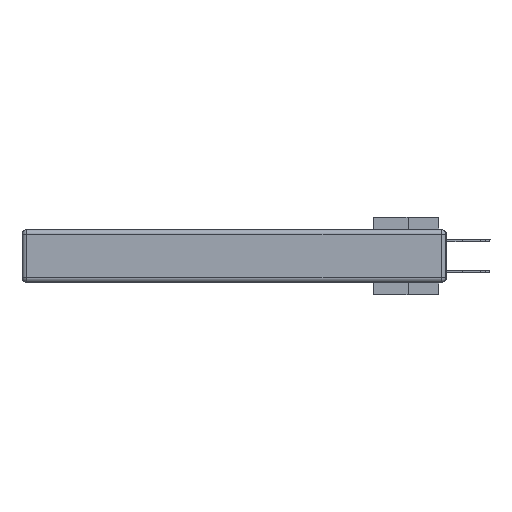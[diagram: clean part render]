
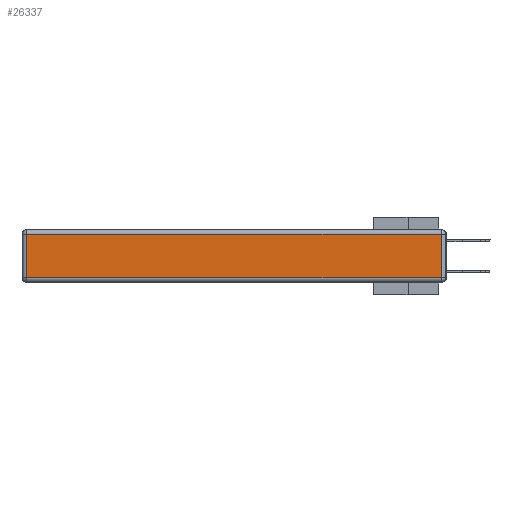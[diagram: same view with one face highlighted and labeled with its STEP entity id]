
A CAD part, left-side view. The second image highlights one B-rep face of the part: STEP entity #26337.
In plain terms, the highlighted planar face has unit normal (-1, 0, 0).
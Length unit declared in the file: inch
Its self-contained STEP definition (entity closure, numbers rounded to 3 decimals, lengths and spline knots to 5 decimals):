
#315 = CARTESIAN_POINT ( 'NONE',  ( 0., 2.72, -0.03 ) ) ;
#1589 = CARTESIAN_POINT ( 'NONE',  ( 0., 0.03, -0.03 ) ) ;
#2590 = ORIENTED_EDGE ( 'NONE', *, *, #18091, .T. ) ;
#4384 = CARTESIAN_POINT ( 'NONE',  ( 0., 0., -0.313 ) ) ;
#4401 = VECTOR ( 'NONE', #8673, 39.37008 ) ;
#5197 = CARTESIAN_POINT ( 'NONE',  ( 0., 0.03, -0.343 ) ) ;
#5312 = DIRECTION ( 'NONE',  ( 0., 1., 0. ) ) ;
#6022 = VECTOR ( 'NONE', #21128, 39.37008 ) ;
#6031 = LINE ( 'NONE', #25385, #21256 ) ;
#6754 = CARTESIAN_POINT ( 'NONE',  ( 0., 0.03, -0.313 ) ) ;
#6885 = LINE ( 'NONE', #4384, #4401 ) ;
#8673 = DIRECTION ( 'NONE',  ( 0., -1., 0. ) ) ;
#8689 = VECTOR ( 'NONE', #17962, 39.37008 ) ;
#9692 = CARTESIAN_POINT ( 'NONE',  ( 0., 0., -0.343 ) ) ;
#10976 = ORIENTED_EDGE ( 'NONE', *, *, #23696, .T. ) ;
#11354 = EDGE_LOOP ( 'NONE', ( #21971, #10976, #28337, #2590 ) ) ;
#13996 = PLANE ( 'NONE',  #22087 ) ;
#15625 = LINE ( 'NONE', #5197, #6022 ) ;
#16360 = DIRECTION ( 'NONE',  ( 0., 0., 1. ) ) ;
#16984 = CARTESIAN_POINT ( 'NONE',  ( 0., 2.72, -0.313 ) ) ;
#17520 = EDGE_CURVE ( 'NONE', #25923, #25482, #6885, .T. ) ;
#17962 = DIRECTION ( 'NONE',  ( 0., 0., -1. ) ) ;
#18091 = EDGE_CURVE ( 'NONE', #28902, #25923, #20392, .T. ) ;
#19339 = FACE_OUTER_BOUND ( 'NONE', #11354, .T. ) ;
#20392 = LINE ( 'NONE', #20502, #8689 ) ;
#20502 = CARTESIAN_POINT ( 'NONE',  ( 0., 2.72, -0.343 ) ) ;
#20504 = EDGE_CURVE ( 'NONE', #26673, #28902, #6031, .T. ) ;
#21128 = DIRECTION ( 'NONE',  ( 0., 0., 1. ) ) ;
#21256 = VECTOR ( 'NONE', #5312, 39.37008 ) ;
#21971 = ORIENTED_EDGE ( 'NONE', *, *, #17520, .T. ) ;
#22087 = AXIS2_PLACEMENT_3D ( 'NONE', #9692, #25108, #16360 ) ;
#23696 = EDGE_CURVE ( 'NONE', #25482, #26673, #15625, .T. ) ;
#25108 = DIRECTION ( 'NONE',  ( -1., 0., 0. ) ) ;
#25385 = CARTESIAN_POINT ( 'NONE',  ( 0., 2.75, -0.03 ) ) ;
#25482 = VERTEX_POINT ( 'NONE', #6754 ) ;
#25923 = VERTEX_POINT ( 'NONE', #16984 ) ;
#26337 = ADVANCED_FACE ( 'NONE', ( #19339 ), #13996, .T. ) ;
#26673 = VERTEX_POINT ( 'NONE', #1589 ) ;
#28337 = ORIENTED_EDGE ( 'NONE', *, *, #20504, .T. ) ;
#28902 = VERTEX_POINT ( 'NONE', #315 ) ;
